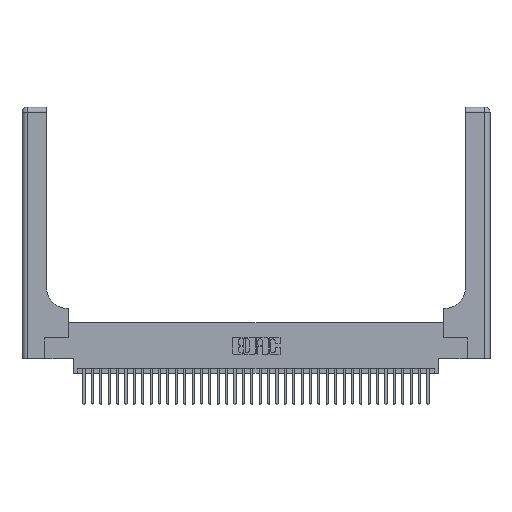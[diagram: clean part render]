
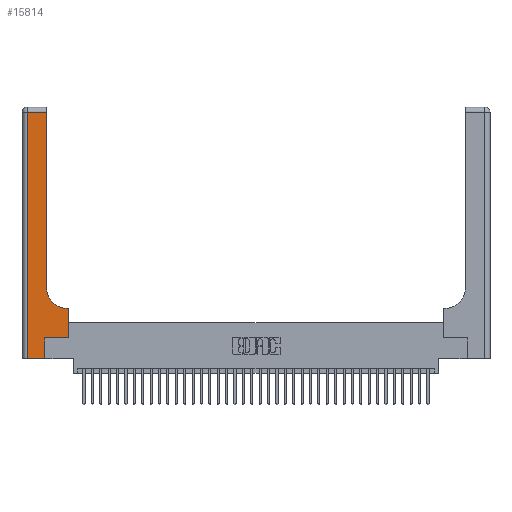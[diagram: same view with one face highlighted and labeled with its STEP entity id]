
A CAD part, top view. The second image highlights one B-rep face of the part: STEP entity #15814.
In plain terms, the highlighted planar face has unit normal (0, 0, 1).
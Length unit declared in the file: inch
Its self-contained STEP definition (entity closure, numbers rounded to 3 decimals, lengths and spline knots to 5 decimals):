
#185 = EDGE_CURVE ( 'NONE', #26945, #15469, #30632, .T. ) ;
#445 = ORIENTED_EDGE ( 'NONE', *, *, #185, .T. ) ;
#861 = VERTEX_POINT ( 'NONE', #23427 ) ;
#1101 = CARTESIAN_POINT ( 'NONE',  ( 0.2915, 2.94, 0.37 ) ) ;
#1563 = EDGE_CURVE ( 'NONE', #861, #26945, #18776, .T. ) ;
#2064 = EDGE_CURVE ( 'NONE', #25451, #22899, #11815, .T. ) ;
#2125 = CARTESIAN_POINT ( 'NONE',  ( 0.2915, 0.85, 0.37 ) ) ;
#5081 = LINE ( 'NONE', #34820, #5991 ) ;
#5230 = ORIENTED_EDGE ( 'NONE', *, *, #19560, .T. ) ;
#5991 = VECTOR ( 'NONE', #14086, 39.37008 ) ;
#6841 = LINE ( 'NONE', #28880, #29515 ) ;
#6969 = DIRECTION ( 'NONE',  ( 1., 0., 0. ) ) ;
#8926 = ORIENTED_EDGE ( 'NONE', *, *, #36230, .T. ) ;
#9168 = ORIENTED_EDGE ( 'NONE', *, *, #16465, .T. ) ;
#10401 = LINE ( 'NONE', #30983, #26115 ) ;
#11531 = CARTESIAN_POINT ( 'NONE',  ( 0.06, 2.94, 0.37 ) ) ;
#11815 = LINE ( 'NONE', #12909, #19699 ) ;
#12090 = LINE ( 'NONE', #33437, #33893 ) ;
#12909 = CARTESIAN_POINT ( 'NONE',  ( 0., 0., 0.37 ) ) ;
#13170 = DIRECTION ( 'NONE',  ( -1., 0., 0. ) ) ;
#13956 = CARTESIAN_POINT ( 'NONE',  ( 0.5415, 0.85, 0.37 ) ) ;
#14004 = PLANE ( 'NONE',  #24914 ) ;
#14086 = DIRECTION ( 'NONE',  ( 0., 1., 0. ) ) ;
#15469 = VERTEX_POINT ( 'NONE', #30340 ) ;
#15814 = ADVANCED_FACE ( 'NONE', ( #19094 ), #14004, .F. ) ;
#16215 = DIRECTION ( 'NONE',  ( 0., -1., 0. ) ) ;
#16465 = EDGE_CURVE ( 'NONE', #23113, #25178, #24676, .T. ) ;
#16935 = DIRECTION ( 'NONE',  ( 1., 0., 0. ) ) ;
#16976 = DIRECTION ( 'NONE',  ( 0., 0., -1. ) ) ;
#17094 = DIRECTION ( 'NONE',  ( -1., 0., 0. ) ) ;
#17484 = AXIS2_PLACEMENT_3D ( 'NONE', #13956, #34697, #16935 ) ;
#17516 = CARTESIAN_POINT ( 'NONE',  ( 0.269, 0., 0.37 ) ) ;
#17754 = EDGE_LOOP ( 'NONE', ( #8926, #24657, #22864, #26087, #25724, #36069, #445, #5230, #9168 ) ) ;
#18638 = DIRECTION ( 'NONE',  ( 0., 1., 0. ) ) ;
#18776 = LINE ( 'NONE', #26458, #26659 ) ;
#19094 = FACE_OUTER_BOUND ( 'NONE', #17754, .T. ) ;
#19560 = EDGE_CURVE ( 'NONE', #15469, #23113, #6841, .T. ) ;
#19699 = VECTOR ( 'NONE', #6969, 39.37008 ) ;
#20659 = DIRECTION ( 'NONE',  ( 1., 0., 0. ) ) ;
#21248 = CARTESIAN_POINT ( 'NONE',  ( 0.06, 0., 0.37 ) ) ;
#22085 = CARTESIAN_POINT ( 'NONE',  ( 0., 2.94, 0.37 ) ) ;
#22864 = ORIENTED_EDGE ( 'NONE', *, *, #34503, .T. ) ;
#22899 = VERTEX_POINT ( 'NONE', #17516 ) ;
#23113 = VERTEX_POINT ( 'NONE', #30183 ) ;
#23427 = CARTESIAN_POINT ( 'NONE',  ( 0.269, 0.25, 0.37 ) ) ;
#24657 = ORIENTED_EDGE ( 'NONE', *, *, #28280, .T. ) ;
#24676 = CIRCLE ( 'NONE', #17484, 0.25 ) ;
#24914 = AXIS2_PLACEMENT_3D ( 'NONE', #34742, #16976, #37708 ) ;
#25178 = VERTEX_POINT ( 'NONE', #2125 ) ;
#25451 = VERTEX_POINT ( 'NONE', #21248 ) ;
#25724 = ORIENTED_EDGE ( 'NONE', *, *, #29017, .T. ) ;
#26087 = ORIENTED_EDGE ( 'NONE', *, *, #2064, .T. ) ;
#26115 = VECTOR ( 'NONE', #16215, 39.37008 ) ;
#26458 = CARTESIAN_POINT ( 'NONE',  ( 0.269, 0.25, 0.37 ) ) ;
#26659 = VECTOR ( 'NONE', #20659, 39.37008 ) ;
#26945 = VERTEX_POINT ( 'NONE', #27730 ) ;
#26954 = VERTEX_POINT ( 'NONE', #1101 ) ;
#27730 = CARTESIAN_POINT ( 'NONE',  ( 0.5585, 0.25, 0.37 ) ) ;
#28280 = EDGE_CURVE ( 'NONE', #26954, #30469, #37072, .T. ) ;
#28380 = CARTESIAN_POINT ( 'NONE',  ( 0.5585, 0.25, 0.37 ) ) ;
#28880 = CARTESIAN_POINT ( 'NONE',  ( 0.2915, 0.6, 0.37 ) ) ;
#29017 = EDGE_CURVE ( 'NONE', #22899, #861, #5081, .T. ) ;
#29175 = VECTOR ( 'NONE', #13170, 39.37008 ) ;
#29515 = VECTOR ( 'NONE', #17094, 39.37008 ) ;
#30183 = CARTESIAN_POINT ( 'NONE',  ( 0.5415, 0.6, 0.37 ) ) ;
#30340 = CARTESIAN_POINT ( 'NONE',  ( 0.5585, 0.6, 0.37 ) ) ;
#30469 = VERTEX_POINT ( 'NONE', #11531 ) ;
#30632 = LINE ( 'NONE', #28380, #37591 ) ;
#30983 = CARTESIAN_POINT ( 'NONE',  ( 0.06, 3., 0.37 ) ) ;
#31399 = DIRECTION ( 'NONE',  ( 0., 1., 0. ) ) ;
#33437 = CARTESIAN_POINT ( 'NONE',  ( 0.2915, 3., 0.37 ) ) ;
#33893 = VECTOR ( 'NONE', #18638, 39.37008 ) ;
#34503 = EDGE_CURVE ( 'NONE', #30469, #25451, #10401, .T. ) ;
#34697 = DIRECTION ( 'NONE',  ( 0., 0., -1. ) ) ;
#34742 = CARTESIAN_POINT ( 'NONE',  ( 0., 3., 0.37 ) ) ;
#34820 = CARTESIAN_POINT ( 'NONE',  ( 0.269, 0., 0.37 ) ) ;
#36069 = ORIENTED_EDGE ( 'NONE', *, *, #1563, .T. ) ;
#36230 = EDGE_CURVE ( 'NONE', #25178, #26954, #12090, .T. ) ;
#37072 = LINE ( 'NONE', #22085, #29175 ) ;
#37591 = VECTOR ( 'NONE', #31399, 39.37008 ) ;
#37708 = DIRECTION ( 'NONE',  ( -1., 0., 0. ) ) ;
